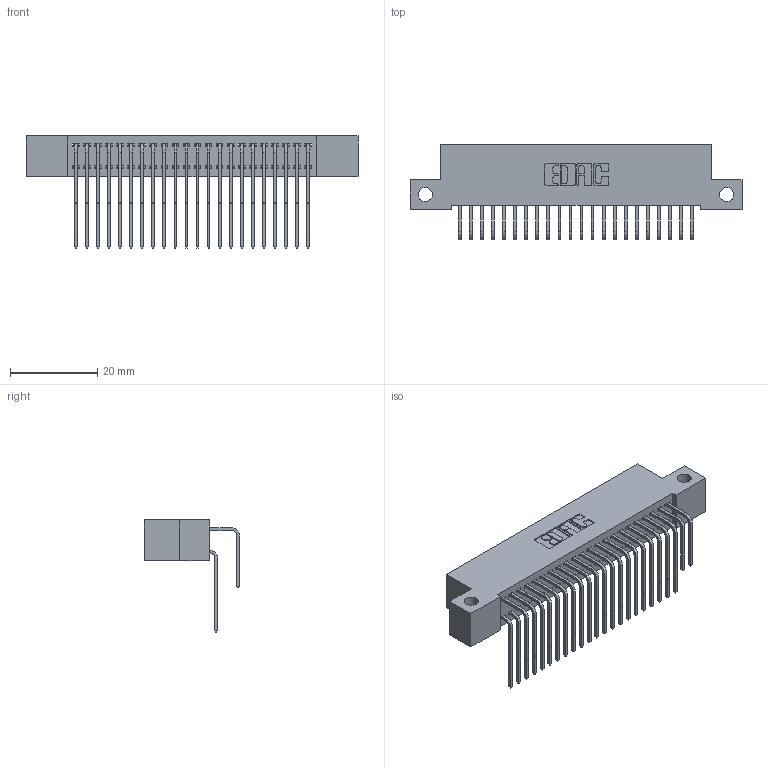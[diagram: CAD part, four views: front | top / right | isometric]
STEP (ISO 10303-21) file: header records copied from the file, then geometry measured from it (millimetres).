
FILE_DESCRIPTION (( 'STEP AP203' ), '1' );
FILE_NAME ('392-044-558-212.STEP', '2019-10-07T22:43:26', ( '' ), ( '' ), 'SwSTEP 2.0', 'SolidWorks 2016', '' );
FILE_SCHEMA (( 'CONFIG_CONTROL_DESIGN' ));
Length unit declared in the file: inch
Products named in the file (4): 342 Part_Side Mount; 345-292-001_558 559 Tail - 1; 345-292-001_558 Tail - 2; 392-044-558-212
Assembly tree (45 placements, depth 2):
  392-044-558-212
    342 Part_Side Mount
    345-292-001_558 559 Tail - 1  x22
    345-292-001_558 Tail - 2  x22
Bounding box: 76.2 x 21.91 x 25.78 mm (x, y, z)
Volume: 6931.8 mm3; surface area: 11778.9 mm2
Topology: 45 solids, 45 shells, 2486 faces, 7383 edges, 4862 vertices
Faces by surface type: plane 1738, cylinder 748
Entity records: 18395 total; most frequent: CARTESIAN_POINT 3121, ORIENTED_EDGE 3006, DIRECTION 2683, EDGE_CURVE 1503, VECTOR 1335, LINE 1335, VERTEX_POINT 998, AXIS2_PLACEMENT_3D 674
